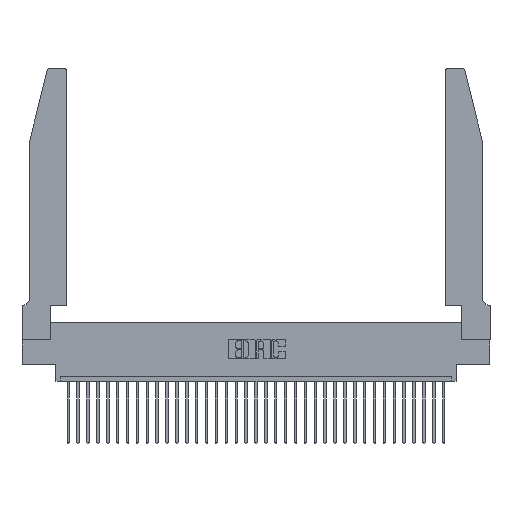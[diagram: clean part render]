
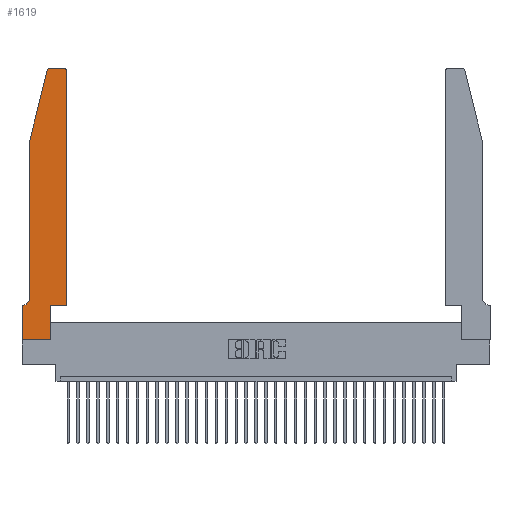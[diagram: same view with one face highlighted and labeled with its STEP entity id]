
A CAD part, top view. The second image highlights one B-rep face of the part: STEP entity #1619.
In plain terms, the highlighted planar face has unit normal (0, 0, 1).
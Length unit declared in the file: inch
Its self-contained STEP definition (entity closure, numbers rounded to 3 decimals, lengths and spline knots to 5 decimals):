
#268 = VERTEX_POINT ( 'NONE', #17135 ) ;
#365 = DIRECTION ( 'NONE',  ( -1., 0., 0. ) ) ;
#994 = AXIS2_PLACEMENT_3D ( 'NONE', #3116, #6167, #21735 ) ;
#1056 = CARTESIAN_POINT ( 'NONE',  ( 0.2865, 0.35, 0.37 ) ) ;
#1404 = VECTOR ( 'NONE', #34583, 39.37008 ) ;
#1601 = EDGE_CURVE ( 'NONE', #25172, #14311, #5171, .T. ) ;
#1619 = ADVANCED_FACE ( 'NONE', ( #13165 ), #13258, .T. ) ;
#1893 = EDGE_CURVE ( 'NONE', #30459, #32536, #13557, .T. ) ;
#2143 = ORIENTED_EDGE ( 'NONE', *, *, #19695, .T. ) ;
#2259 = EDGE_CURVE ( 'NONE', #13669, #33075, #17301, .T. ) ;
#3116 = CARTESIAN_POINT ( 'NONE',  ( 0.4205, 2.72, 0.37 ) ) ;
#3762 = AXIS2_PLACEMENT_3D ( 'NONE', #7642, #15736, #26213 ) ;
#3932 = VECTOR ( 'NONE', #7804, 39.37008 ) ;
#4292 = EDGE_CURVE ( 'NONE', #5419, #25172, #14556, .T. ) ;
#4296 = EDGE_CURVE ( 'NONE', #28523, #10768, #13674, .T. ) ;
#4596 = ORIENTED_EDGE ( 'NONE', *, *, #2259, .T. ) ;
#4613 = EDGE_CURVE ( 'NONE', #14311, #28523, #17831, .T. ) ;
#4939 = EDGE_CURVE ( 'NONE', #10768, #18605, #32919, .T. ) ;
#5169 = CARTESIAN_POINT ( 'NONE',  ( 0.4205, 2.75, 0.37 ) ) ;
#5171 = LINE ( 'NONE', #5868, #10609 ) ;
#5419 = VERTEX_POINT ( 'NONE', #28602 ) ;
#5868 = CARTESIAN_POINT ( 'NONE',  ( 0.0755, 0.35, 0.37 ) ) ;
#5938 = EDGE_CURVE ( 'NONE', #18605, #30459, #27353, .T. ) ;
#6167 = DIRECTION ( 'NONE',  ( 0., 0., 1. ) ) ;
#7642 = CARTESIAN_POINT ( 'NONE',  ( 0.284, 2.72, 0.37 ) ) ;
#7804 = DIRECTION ( 'NONE',  ( 1., 0., 0. ) ) ;
#8199 = CARTESIAN_POINT ( 'NONE',  ( 0., 0., 0.37 ) ) ;
#8874 = ORIENTED_EDGE ( 'NONE', *, *, #1601, .T. ) ;
#8998 = CARTESIAN_POINT ( 'NONE',  ( 0.2865, 0.35, 0.37 ) ) ;
#9940 = EDGE_CURVE ( 'NONE', #32807, #5419, #14751, .T. ) ;
#10609 = VECTOR ( 'NONE', #24121, 39.37008 ) ;
#10664 = VECTOR ( 'NONE', #33032, 39.37008 ) ;
#10768 = VERTEX_POINT ( 'NONE', #14804 ) ;
#11339 = CARTESIAN_POINT ( 'NONE',  ( 0.2605, 2.75, 0.37 ) ) ;
#11467 = CARTESIAN_POINT ( 'NONE',  ( 0.0055, 0.35, 0.37 ) ) ;
#11829 = DIRECTION ( 'NONE',  ( 0., 0., -1. ) ) ;
#12182 = VECTOR ( 'NONE', #24189, 39.37008 ) ;
#12771 = CARTESIAN_POINT ( 'NONE',  ( 0.4505, 0.35, 0.37 ) ) ;
#13165 = FACE_OUTER_BOUND ( 'NONE', #17786, .T. ) ;
#13258 = PLANE ( 'NONE',  #27244 ) ;
#13374 = DIRECTION ( 'NONE',  ( 1., 0., 0. ) ) ;
#13557 = LINE ( 'NONE', #13608, #1404 ) ;
#13608 = CARTESIAN_POINT ( 'NONE',  ( 0.4505, 0.35, 0.37 ) ) ;
#13669 = VERTEX_POINT ( 'NONE', #5169 ) ;
#13674 = LINE ( 'NONE', #8199, #19095 ) ;
#13698 = ORIENTED_EDGE ( 'NONE', *, *, #9940, .T. ) ;
#14311 = VERTEX_POINT ( 'NONE', #20663 ) ;
#14556 = CIRCLE ( 'NONE', #25724, 0.07 ) ;
#14751 = LINE ( 'NONE', #34428, #12182 ) ;
#14804 = CARTESIAN_POINT ( 'NONE',  ( 0.2865, 0., 0.37 ) ) ;
#15036 = CIRCLE ( 'NONE', #3762, 0.03 ) ;
#15313 = DIRECTION ( 'NONE',  ( 0., -1., 0. ) ) ;
#15630 = ORIENTED_EDGE ( 'NONE', *, *, #1893, .T. ) ;
#15713 = ORIENTED_EDGE ( 'NONE', *, *, #4296, .T. ) ;
#15736 = DIRECTION ( 'NONE',  ( 0., 0., 1. ) ) ;
#15902 = CARTESIAN_POINT ( 'NONE',  ( 0.4505, 0.35, 0.37 ) ) ;
#16431 = EDGE_CURVE ( 'NONE', #268, #32807, #33851, .T. ) ;
#17135 = CARTESIAN_POINT ( 'NONE',  ( 0.25487, 2.72718, 0.37 ) ) ;
#17301 = LINE ( 'NONE', #11339, #29014 ) ;
#17786 = EDGE_LOOP ( 'NONE', ( #4596, #20203, #33621, #13698, #19299, #8874, #18964, #15713, #18933, #30226, #15630, #2143 ) ) ;
#17831 = LINE ( 'NONE', #26362, #19509 ) ;
#18605 = VERTEX_POINT ( 'NONE', #1056 ) ;
#18933 = ORIENTED_EDGE ( 'NONE', *, *, #4939, .T. ) ;
#18964 = ORIENTED_EDGE ( 'NONE', *, *, #4613, .T. ) ;
#19095 = VECTOR ( 'NONE', #34580, 39.37008 ) ;
#19299 = ORIENTED_EDGE ( 'NONE', *, *, #4292, .T. ) ;
#19509 = VECTOR ( 'NONE', #15313, 39.37008 ) ;
#19695 = EDGE_CURVE ( 'NONE', #32536, #13669, #21238, .T. ) ;
#20203 = ORIENTED_EDGE ( 'NONE', *, *, #23729, .T. ) ;
#20355 = CARTESIAN_POINT ( 'NONE',  ( 0.0755, 2., 0.37 ) ) ;
#20663 = CARTESIAN_POINT ( 'NONE',  ( 0., 0.35, 0.37 ) ) ;
#21238 = CIRCLE ( 'NONE', #994, 0.03 ) ;
#21366 = CARTESIAN_POINT ( 'NONE',  ( 0.284, 2.75, 0.37 ) ) ;
#21735 = DIRECTION ( 'NONE',  ( 1., 0., 0. ) ) ;
#23729 = EDGE_CURVE ( 'NONE', #33075, #268, #15036, .T. ) ;
#24121 = DIRECTION ( 'NONE',  ( -1., 0., 0. ) ) ;
#24189 = DIRECTION ( 'NONE',  ( 0., -1., 0. ) ) ;
#24368 = CARTESIAN_POINT ( 'NONE',  ( 0., 0., 0.37 ) ) ;
#25068 = DIRECTION ( 'NONE',  ( -0.239, -0.971, 0. ) ) ;
#25172 = VERTEX_POINT ( 'NONE', #11467 ) ;
#25724 = AXIS2_PLACEMENT_3D ( 'NONE', #30578, #11829, #365 ) ;
#26213 = DIRECTION ( 'NONE',  ( 1., 0., 0. ) ) ;
#26362 = CARTESIAN_POINT ( 'NONE',  ( 0., 0., 0.37 ) ) ;
#27244 = AXIS2_PLACEMENT_3D ( 'NONE', #29722, #31959, #13374 ) ;
#27353 = LINE ( 'NONE', #15902, #3932 ) ;
#28523 = VERTEX_POINT ( 'NONE', #24368 ) ;
#28602 = CARTESIAN_POINT ( 'NONE',  ( 0.0755, 0.42, 0.37 ) ) ;
#29014 = VECTOR ( 'NONE', #32302, 39.37008 ) ;
#29722 = CARTESIAN_POINT ( 'NONE',  ( 0., 0.35, 0.37 ) ) ;
#30226 = ORIENTED_EDGE ( 'NONE', *, *, #5938, .T. ) ;
#30459 = VERTEX_POINT ( 'NONE', #12771 ) ;
#30578 = CARTESIAN_POINT ( 'NONE',  ( 0.0055, 0.42, 0.37 ) ) ;
#30898 = VECTOR ( 'NONE', #25068, 39.37008 ) ;
#31959 = DIRECTION ( 'NONE',  ( 0., 0., 1. ) ) ;
#32223 = CARTESIAN_POINT ( 'NONE',  ( 0.0755, 2., 0.37 ) ) ;
#32302 = DIRECTION ( 'NONE',  ( -1., 0., 0. ) ) ;
#32536 = VERTEX_POINT ( 'NONE', #32635 ) ;
#32635 = CARTESIAN_POINT ( 'NONE',  ( 0.4505, 2.72, 0.37 ) ) ;
#32807 = VERTEX_POINT ( 'NONE', #20355 ) ;
#32919 = LINE ( 'NONE', #8998, #10664 ) ;
#33032 = DIRECTION ( 'NONE',  ( 0., 1., 0. ) ) ;
#33075 = VERTEX_POINT ( 'NONE', #21366 ) ;
#33621 = ORIENTED_EDGE ( 'NONE', *, *, #16431, .T. ) ;
#33851 = LINE ( 'NONE', #32223, #30898 ) ;
#34428 = CARTESIAN_POINT ( 'NONE',  ( 0.0755, 2., 0.37 ) ) ;
#34580 = DIRECTION ( 'NONE',  ( 1., 0., 0. ) ) ;
#34583 = DIRECTION ( 'NONE',  ( 0., 1., 0. ) ) ;
